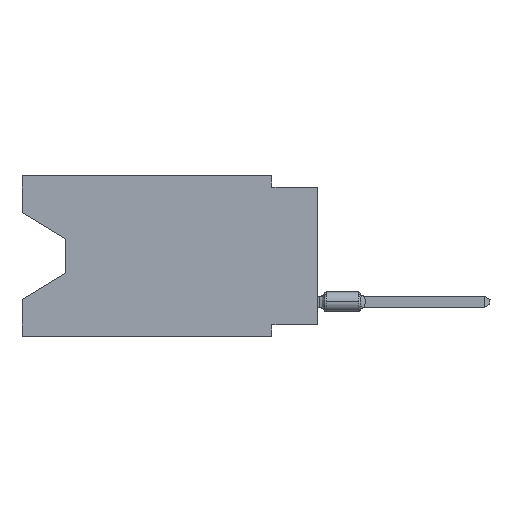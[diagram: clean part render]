
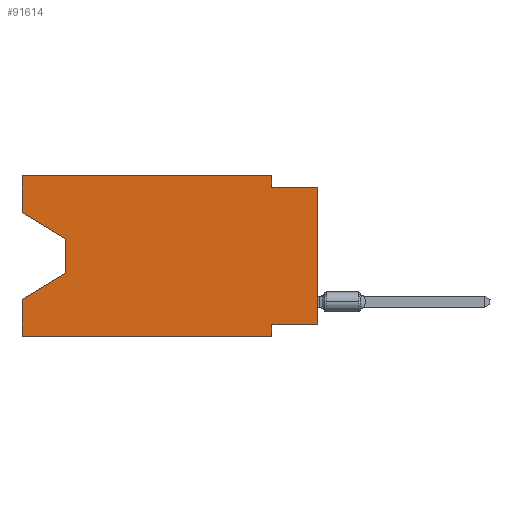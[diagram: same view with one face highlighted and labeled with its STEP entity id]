
A CAD part, left-side view. The second image highlights one B-rep face of the part: STEP entity #91614.
In plain terms, the highlighted planar face has unit normal (-1, 0, 0).
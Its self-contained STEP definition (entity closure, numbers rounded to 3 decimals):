
#1266 = VERTEX_POINT ( 'NONE', #109190 ) ;
#3472 = CARTESIAN_POINT ( 'NONE',  ( 0., 2.54, -8.255 ) ) ;
#3909 = CARTESIAN_POINT ( 'NONE',  ( 0., 0., -0.635 ) ) ;
#4127 = VERTEX_POINT ( 'NONE', #82753 ) ;
#4853 = VERTEX_POINT ( 'NONE', #13229 ) ;
#6089 = VECTOR ( 'NONE', #52469, 1000. ) ;
#6147 = CARTESIAN_POINT ( 'NONE',  ( 0., 2.54, -0.635 ) ) ;
#7213 = ORIENTED_EDGE ( 'NONE', *, *, #112478, .T. ) ;
#7401 = DIRECTION ( 'NONE',  ( 0., -1., 0. ) ) ;
#7758 = ORIENTED_EDGE ( 'NONE', *, *, #102229, .F. ) ;
#8943 = ORIENTED_EDGE ( 'NONE', *, *, #76400, .T. ) ;
#9693 = PLANE ( 'NONE',  #102328 ) ;
#10558 = VERTEX_POINT ( 'NONE', #3472 ) ;
#13229 = CARTESIAN_POINT ( 'NONE',  ( 0., 2.54, 0. ) ) ;
#13649 = VECTOR ( 'NONE', #110970, 1000. ) ;
#14067 = VERTEX_POINT ( 'NONE', #16580 ) ;
#16580 = CARTESIAN_POINT ( 'NONE',  ( 0., 2.54, -8.89 ) ) ;
#16785 = CARTESIAN_POINT ( 'NONE',  ( 0., 16.383, 0. ) ) ;
#22076 = ORIENTED_EDGE ( 'NONE', *, *, #104229, .F. ) ;
#22346 = VECTOR ( 'NONE', #41515, 1000. ) ;
#22419 = EDGE_CURVE ( 'NONE', #10558, #14067, #48772, .T. ) ;
#22725 = CARTESIAN_POINT ( 'NONE',  ( 0., 13.97, -5.385 ) ) ;
#23160 = VECTOR ( 'NONE', #38656, 1000. ) ;
#23568 = DIRECTION ( 'NONE',  ( 0., 0., -1. ) ) ;
#28684 = CARTESIAN_POINT ( 'NONE',  ( 0., 0., -0.635 ) ) ;
#30403 = VECTOR ( 'NONE', #102408, 1000. ) ;
#33884 = LINE ( 'NONE', #42688, #71186 ) ;
#33920 = LINE ( 'NONE', #69776, #104351 ) ;
#36441 = EDGE_CURVE ( 'NONE', #48149, #43246, #77928, .T. ) ;
#37007 = ORIENTED_EDGE ( 'NONE', *, *, #88088, .T. ) ;
#37849 = CARTESIAN_POINT ( 'NONE',  ( 0., 16.383, -2.038 ) ) ;
#38656 = DIRECTION ( 'NONE',  ( 0., -1., 0. ) ) ;
#39047 = VECTOR ( 'NONE', #95001, 1000. ) ;
#41515 = DIRECTION ( 'NONE',  ( 0., 0.855, -0.519 ) ) ;
#42688 = CARTESIAN_POINT ( 'NONE',  ( 0., 16.383, -8.89 ) ) ;
#43246 = VERTEX_POINT ( 'NONE', #44089 ) ;
#44089 = CARTESIAN_POINT ( 'NONE',  ( 0., 16.383, 0. ) ) ;
#44230 = CARTESIAN_POINT ( 'NONE',  ( 0., 16.383, 0. ) ) ;
#45378 = LINE ( 'NONE', #44230, #6089 ) ;
#46950 = CARTESIAN_POINT ( 'NONE',  ( 0., 13.97, -5.385 ) ) ;
#48149 = VERTEX_POINT ( 'NONE', #37849 ) ;
#48772 = LINE ( 'NONE', #101139, #81206 ) ;
#50797 = ORIENTED_EDGE ( 'NONE', *, *, #112097, .T. ) ;
#50964 = ORIENTED_EDGE ( 'NONE', *, *, #36441, .F. ) ;
#52469 = DIRECTION ( 'NONE',  ( 0., -1., 0. ) ) ;
#52652 = DIRECTION ( 'NONE',  ( 0., 0., -1. ) ) ;
#58078 = VERTEX_POINT ( 'NONE', #46950 ) ;
#58587 = LINE ( 'NONE', #3909, #23160 ) ;
#59433 = CARTESIAN_POINT ( 'NONE',  ( 0., 13.97, -3.505 ) ) ;
#60729 = EDGE_CURVE ( 'NONE', #1266, #10558, #33920, .T. ) ;
#60795 = LINE ( 'NONE', #97260, #110641 ) ;
#63237 = DIRECTION ( 'NONE',  ( 1., 0., 0. ) ) ;
#63770 = VERTEX_POINT ( 'NONE', #77994 ) ;
#64107 = DIRECTION ( 'NONE',  ( 0., 0., -1. ) ) ;
#66598 = VERTEX_POINT ( 'NONE', #6147 ) ;
#67090 = CARTESIAN_POINT ( 'NONE',  ( 0., 2.54, 0. ) ) ;
#68491 = CARTESIAN_POINT ( 'NONE',  ( 0., 16.383, 0. ) ) ;
#69667 = ORIENTED_EDGE ( 'NONE', *, *, #87766, .T. ) ;
#69776 = CARTESIAN_POINT ( 'NONE',  ( 0., 0., -8.255 ) ) ;
#70382 = DIRECTION ( 'NONE',  ( 0., 1., 0. ) ) ;
#71033 = ORIENTED_EDGE ( 'NONE', *, *, #116098, .F. ) ;
#71113 = ORIENTED_EDGE ( 'NONE', *, *, #60729, .F. ) ;
#71186 = VECTOR ( 'NONE', #7401, 1000. ) ;
#73680 = ORIENTED_EDGE ( 'NONE', *, *, #101088, .F. ) ;
#76400 = EDGE_CURVE ( 'NONE', #58078, #4127, #78554, .T. ) ;
#77928 = LINE ( 'NONE', #102688, #39047 ) ;
#77994 = CARTESIAN_POINT ( 'NONE',  ( 0., 16.383, -8.89 ) ) ;
#78554 = LINE ( 'NONE', #22725, #22346 ) ;
#81206 = VECTOR ( 'NONE', #64107, 1000. ) ;
#82753 = CARTESIAN_POINT ( 'NONE',  ( 0., 16.383, -6.852 ) ) ;
#84491 = LINE ( 'NONE', #102165, #13649 ) ;
#86472 = LINE ( 'NONE', #59433, #114005 ) ;
#87766 = EDGE_CURVE ( 'NONE', #103263, #58078, #86472, .T. ) ;
#88088 = EDGE_CURVE ( 'NONE', #48149, #103263, #84491, .T. ) ;
#90129 = CARTESIAN_POINT ( 'NONE',  ( 0., 13.97, -3.505 ) ) ;
#91614 = ADVANCED_FACE ( 'NONE', ( #106188 ), #9693, .F. ) ;
#92457 = VERTEX_POINT ( 'NONE', #28684 ) ;
#92554 = EDGE_LOOP ( 'NONE', ( #37007, #69667, #8943, #71033, #50797, #110910, #71113, #7213, #22076, #7758, #73680, #50964 ) ) ;
#93828 = LINE ( 'NONE', #68491, #115787 ) ;
#95001 = DIRECTION ( 'NONE',  ( 0., 0., 1. ) ) ;
#95284 = LINE ( 'NONE', #67090, #30403 ) ;
#97260 = CARTESIAN_POINT ( 'NONE',  ( 0., 0., 0. ) ) ;
#101088 = EDGE_CURVE ( 'NONE', #43246, #4853, #45378, .T. ) ;
#101139 = CARTESIAN_POINT ( 'NONE',  ( 0., 2.54, -8.89 ) ) ;
#102165 = CARTESIAN_POINT ( 'NONE',  ( 0., 16.383, -2.038 ) ) ;
#102229 = EDGE_CURVE ( 'NONE', #4853, #66598, #95284, .T. ) ;
#102328 = AXIS2_PLACEMENT_3D ( 'NONE', #16785, #63237, #52652 ) ;
#102408 = DIRECTION ( 'NONE',  ( 0., 0., -1. ) ) ;
#102688 = CARTESIAN_POINT ( 'NONE',  ( 0., 16.383, 0. ) ) ;
#103263 = VERTEX_POINT ( 'NONE', #90129 ) ;
#104229 = EDGE_CURVE ( 'NONE', #66598, #92457, #58587, .T. ) ;
#104351 = VECTOR ( 'NONE', #70382, 1000. ) ;
#104373 = DIRECTION ( 'NONE',  ( 0., 0., 1. ) ) ;
#106188 = FACE_OUTER_BOUND ( 'NONE', #92554, .T. ) ;
#109190 = CARTESIAN_POINT ( 'NONE',  ( 0., 0., -8.255 ) ) ;
#110641 = VECTOR ( 'NONE', #115496, 1000. ) ;
#110910 = ORIENTED_EDGE ( 'NONE', *, *, #22419, .F. ) ;
#110970 = DIRECTION ( 'NONE',  ( 0., -0.855, -0.519 ) ) ;
#112097 = EDGE_CURVE ( 'NONE', #63770, #14067, #33884, .T. ) ;
#112478 = EDGE_CURVE ( 'NONE', #1266, #92457, #60795, .T. ) ;
#114005 = VECTOR ( 'NONE', #23568, 1000. ) ;
#115496 = DIRECTION ( 'NONE',  ( 0., 0., 1. ) ) ;
#115787 = VECTOR ( 'NONE', #104373, 1000. ) ;
#116098 = EDGE_CURVE ( 'NONE', #63770, #4127, #93828, .T. ) ;
